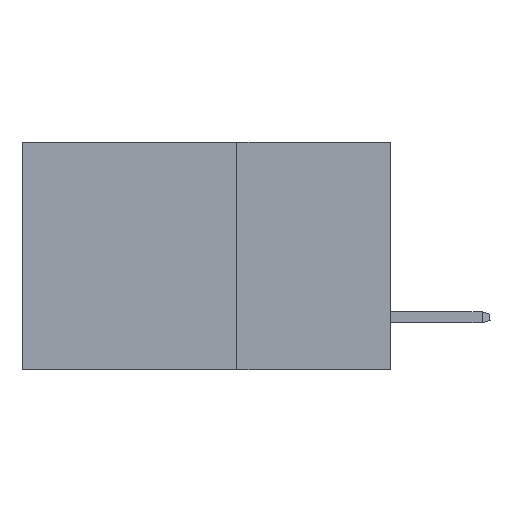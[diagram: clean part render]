
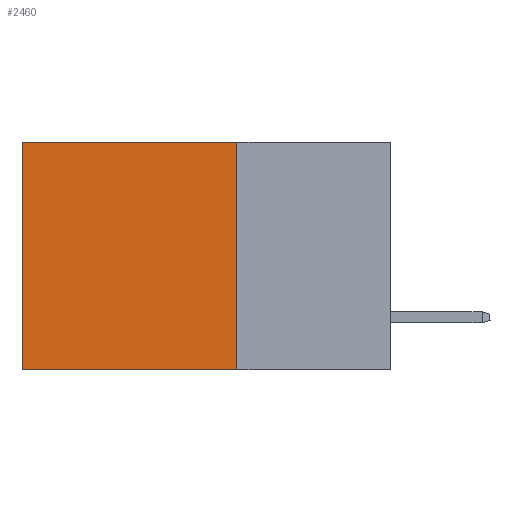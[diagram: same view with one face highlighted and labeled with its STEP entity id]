
A CAD part, left-side view. The second image highlights one B-rep face of the part: STEP entity #2460.
In plain terms, the highlighted planar face has unit normal (-1, 0, 0).
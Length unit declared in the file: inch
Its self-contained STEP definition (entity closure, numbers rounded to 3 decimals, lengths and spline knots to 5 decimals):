
#540 = DIRECTION ( 'NONE',  ( 1., 0., 0. ) ) ;
#790 = CARTESIAN_POINT ( 'NONE',  ( 0.2875, 0.6, 0. ) ) ;
#931 = AXIS2_PLACEMENT_3D ( 'NONE', #15170, #540, #25430 ) ;
#1289 = EDGE_LOOP ( 'NONE', ( #1678, #12354, #16718, #18906 ) ) ;
#1552 = VECTOR ( 'NONE', #1692, 39.37008 ) ;
#1678 = ORIENTED_EDGE ( 'NONE', *, *, #15473, .T. ) ;
#1692 = DIRECTION ( 'NONE',  ( 0., 1., 0. ) ) ;
#2340 = VECTOR ( 'NONE', #22109, 39.37008 ) ;
#2460 = ADVANCED_FACE ( 'NONE', ( #24043 ), #25146, .F. ) ;
#3489 = LINE ( 'NONE', #18501, #1552 ) ;
#6154 = VECTOR ( 'NONE', #23518, 39.37008 ) ;
#7184 = CARTESIAN_POINT ( 'NONE',  ( 0.2875, 0.25, 0. ) ) ;
#10292 = CARTESIAN_POINT ( 'NONE',  ( 0.2875, 0.25, -0.37 ) ) ;
#10682 = DIRECTION ( 'NONE',  ( 0., 0., -1. ) ) ;
#11277 = CARTESIAN_POINT ( 'NONE',  ( 0.2875, 0.6, -0.37 ) ) ;
#11840 = VERTEX_POINT ( 'NONE', #14971 ) ;
#12354 = ORIENTED_EDGE ( 'NONE', *, *, #14057, .F. ) ;
#13081 = VERTEX_POINT ( 'NONE', #11277 ) ;
#14057 = EDGE_CURVE ( 'NONE', #16854, #13081, #19183, .T. ) ;
#14971 = CARTESIAN_POINT ( 'NONE',  ( 0.2875, 0.6, 0. ) ) ;
#15170 = CARTESIAN_POINT ( 'NONE',  ( 0.2875, 0.25, 0. ) ) ;
#15473 = EDGE_CURVE ( 'NONE', #11840, #13081, #23260, .T. ) ;
#16718 = ORIENTED_EDGE ( 'NONE', *, *, #18102, .F. ) ;
#16854 = VERTEX_POINT ( 'NONE', #10292 ) ;
#18102 = EDGE_CURVE ( 'NONE', #18833, #16854, #19611, .T. ) ;
#18501 = CARTESIAN_POINT ( 'NONE',  ( 0.2875, 0.25, 0. ) ) ;
#18833 = VERTEX_POINT ( 'NONE', #7184 ) ;
#18906 = ORIENTED_EDGE ( 'NONE', *, *, #19998, .T. ) ;
#19183 = LINE ( 'NONE', #20109, #2340 ) ;
#19611 = LINE ( 'NONE', #23030, #22822 ) ;
#19998 = EDGE_CURVE ( 'NONE', #18833, #11840, #3489, .T. ) ;
#20109 = CARTESIAN_POINT ( 'NONE',  ( 0.2875, 0.25, -0.37 ) ) ;
#22109 = DIRECTION ( 'NONE',  ( 0., 1., 0. ) ) ;
#22822 = VECTOR ( 'NONE', #10682, 39.37008 ) ;
#23030 = CARTESIAN_POINT ( 'NONE',  ( 0.2875, 0.25, 0. ) ) ;
#23260 = LINE ( 'NONE', #790, #6154 ) ;
#23518 = DIRECTION ( 'NONE',  ( 0., 0., -1. ) ) ;
#24043 = FACE_OUTER_BOUND ( 'NONE', #1289, .T. ) ;
#25146 = PLANE ( 'NONE',  #931 ) ;
#25430 = DIRECTION ( 'NONE',  ( 0., 0., -1. ) ) ;
